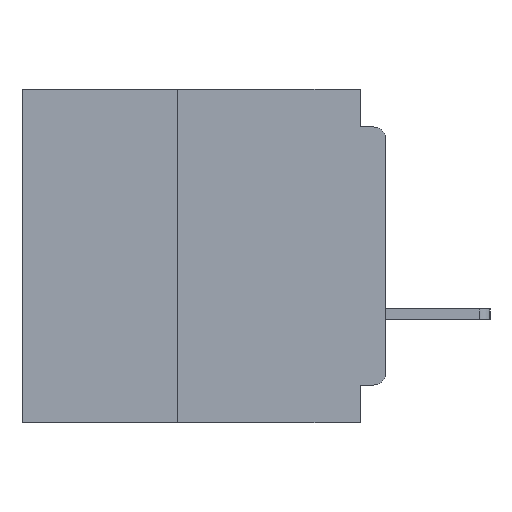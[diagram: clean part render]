
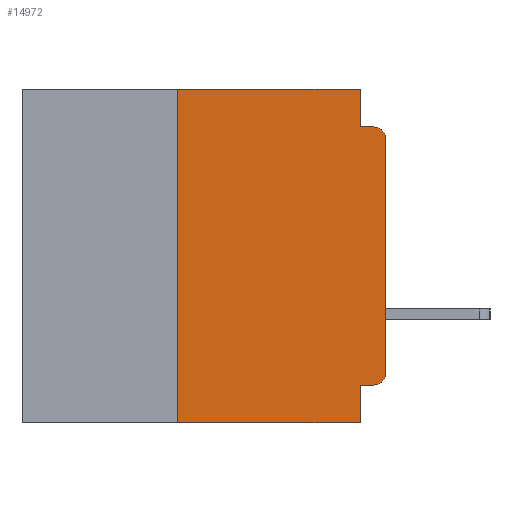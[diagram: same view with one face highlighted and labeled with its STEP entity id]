
A CAD part, left-side view. The second image highlights one B-rep face of the part: STEP entity #14972.
In plain terms, the highlighted planar face has unit normal (-1, 0, 0).
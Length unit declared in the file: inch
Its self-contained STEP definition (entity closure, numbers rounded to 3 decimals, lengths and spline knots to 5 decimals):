
#317 = ORIENTED_EDGE ( 'NONE', *, *, #792, .F. ) ;
#404 = CARTESIAN_POINT ( 'NONE',  ( 0., 0., -0.045 ) ) ;
#477 = LINE ( 'NONE', #39365, #16300 ) ;
#792 = EDGE_CURVE ( 'NONE', #34249, #23043, #32189, .T. ) ;
#835 = LINE ( 'NONE', #26741, #16669 ) ;
#1063 = ORIENTED_EDGE ( 'NONE', *, *, #35145, .T. ) ;
#1372 = LINE ( 'NONE', #39478, #8784 ) ;
#1627 = CARTESIAN_POINT ( 'NONE',  ( 0., 0.25, -0.4 ) ) ;
#2111 = DIRECTION ( 'NONE',  ( 0., 0., -1. ) ) ;
#2908 = EDGE_CURVE ( 'NONE', #33924, #28827, #24180, .T. ) ;
#3327 = CARTESIAN_POINT ( 'NONE',  ( 0., 0.031, -0.045 ) ) ;
#3510 = EDGE_CURVE ( 'NONE', #23043, #33924, #477, .T. ) ;
#3692 = ORIENTED_EDGE ( 'NONE', *, *, #33052, .F. ) ;
#4045 = ORIENTED_EDGE ( 'NONE', *, *, #2908, .F. ) ;
#4411 = DIRECTION ( 'NONE',  ( 1., 0., 0. ) ) ;
#4906 = DIRECTION ( 'NONE',  ( 0., 0., -1. ) ) ;
#4947 = ORIENTED_EDGE ( 'NONE', *, *, #22686, .F. ) ;
#4999 = EDGE_CURVE ( 'NONE', #9444, #7783, #835, .T. ) ;
#5172 = EDGE_LOOP ( 'NONE', ( #27229, #22282, #9449, #4045, #31001, #317, #1063, #3692, #4947, #5655 ) ) ;
#5655 = ORIENTED_EDGE ( 'NONE', *, *, #37965, .T. ) ;
#5801 = EDGE_CURVE ( 'NONE', #7783, #9494, #13127, .T. ) ;
#6443 = LINE ( 'NONE', #23766, #39601 ) ;
#7588 = CARTESIAN_POINT ( 'NONE',  ( 0., 0.031, -0.355 ) ) ;
#7783 = VERTEX_POINT ( 'NONE', #21004 ) ;
#8784 = VECTOR ( 'NONE', #24107, 39.37008 ) ;
#9444 = VERTEX_POINT ( 'NONE', #35533 ) ;
#9449 = ORIENTED_EDGE ( 'NONE', *, *, #37206, .F. ) ;
#9494 = VERTEX_POINT ( 'NONE', #26444 ) ;
#9513 = DIRECTION ( 'NONE',  ( 0., 0., -1. ) ) ;
#9569 = DIRECTION ( 'NONE',  ( -1., 0., 0. ) ) ;
#9646 = CARTESIAN_POINT ( 'NONE',  ( 0., 0.015, -0.06 ) ) ;
#12024 = VECTOR ( 'NONE', #18635, 39.37008 ) ;
#13127 = CIRCLE ( 'NONE', #31725, 0.015 ) ;
#14162 = CARTESIAN_POINT ( 'NONE',  ( 0., 0.25, 0. ) ) ;
#14673 = AXIS2_PLACEMENT_3D ( 'NONE', #23292, #4411, #26365 ) ;
#14972 = ADVANCED_FACE ( 'NONE', ( #22209 ), #35587, .F. ) ;
#15386 = VERTEX_POINT ( 'NONE', #32702 ) ;
#15880 = VECTOR ( 'NONE', #22164, 39.37008 ) ;
#16168 = DIRECTION ( 'NONE',  ( 0., -1., 0. ) ) ;
#16300 = VECTOR ( 'NONE', #39157, 39.37008 ) ;
#16549 = DIRECTION ( 'NONE',  ( 0., 0., 1. ) ) ;
#16669 = VECTOR ( 'NONE', #26215, 39.37008 ) ;
#18253 = CARTESIAN_POINT ( 'NONE',  ( 0., 0.015, -0.355 ) ) ;
#18635 = DIRECTION ( 'NONE',  ( 0., 1., 0. ) ) ;
#20461 = LINE ( 'NONE', #30924, #12024 ) ;
#21004 = CARTESIAN_POINT ( 'NONE',  ( 0., 0., -0.06 ) ) ;
#21076 = DIRECTION ( 'NONE',  ( -1., 0., 0. ) ) ;
#22164 = DIRECTION ( 'NONE',  ( 0., 0., -1. ) ) ;
#22209 = FACE_OUTER_BOUND ( 'NONE', #5172, .T. ) ;
#22282 = ORIENTED_EDGE ( 'NONE', *, *, #5801, .T. ) ;
#22686 = EDGE_CURVE ( 'NONE', #29262, #24522, #20461, .T. ) ;
#23043 = VERTEX_POINT ( 'NONE', #14162 ) ;
#23167 = CARTESIAN_POINT ( 'NONE',  ( 0., 0.031, 0. ) ) ;
#23292 = CARTESIAN_POINT ( 'NONE',  ( 0., 0.437, 0. ) ) ;
#23766 = CARTESIAN_POINT ( 'NONE',  ( 0., 0.031, -0.4 ) ) ;
#24107 = DIRECTION ( 'NONE',  ( 0., -1., 0. ) ) ;
#24180 = LINE ( 'NONE', #23167, #15880 ) ;
#24522 = VERTEX_POINT ( 'NONE', #7588 ) ;
#26215 = DIRECTION ( 'NONE',  ( 0., 0., 1. ) ) ;
#26365 = DIRECTION ( 'NONE',  ( 0., 0., -1. ) ) ;
#26444 = CARTESIAN_POINT ( 'NONE',  ( 0., 0.015, -0.045 ) ) ;
#26741 = CARTESIAN_POINT ( 'NONE',  ( 0., 0., 0. ) ) ;
#27229 = ORIENTED_EDGE ( 'NONE', *, *, #4999, .T. ) ;
#27823 = AXIS2_PLACEMENT_3D ( 'NONE', #39505, #21076, #2111 ) ;
#28827 = VERTEX_POINT ( 'NONE', #3327 ) ;
#29262 = VERTEX_POINT ( 'NONE', #18253 ) ;
#29907 = CARTESIAN_POINT ( 'NONE',  ( 0., 0.25, -0.4 ) ) ;
#30536 = VECTOR ( 'NONE', #16168, 39.37008 ) ;
#30924 = CARTESIAN_POINT ( 'NONE',  ( 0., 0., -0.355 ) ) ;
#31001 = ORIENTED_EDGE ( 'NONE', *, *, #3510, .F. ) ;
#31240 = VECTOR ( 'NONE', #16549, 39.37008 ) ;
#31725 = AXIS2_PLACEMENT_3D ( 'NONE', #9646, #9569, #9513 ) ;
#32189 = LINE ( 'NONE', #1627, #31240 ) ;
#32702 = CARTESIAN_POINT ( 'NONE',  ( 0., 0.031, -0.4 ) ) ;
#33052 = EDGE_CURVE ( 'NONE', #24522, #15386, #6443, .T. ) ;
#33923 = CIRCLE ( 'NONE', #27823, 0.015 ) ;
#33924 = VERTEX_POINT ( 'NONE', #40155 ) ;
#34249 = VERTEX_POINT ( 'NONE', #29907 ) ;
#35145 = EDGE_CURVE ( 'NONE', #34249, #15386, #1372, .T. ) ;
#35533 = CARTESIAN_POINT ( 'NONE',  ( 0., 0., -0.34 ) ) ;
#35587 = PLANE ( 'NONE',  #14673 ) ;
#37206 = EDGE_CURVE ( 'NONE', #28827, #9494, #39691, .T. ) ;
#37965 = EDGE_CURVE ( 'NONE', #29262, #9444, #33923, .T. ) ;
#39157 = DIRECTION ( 'NONE',  ( 0., -1., 0. ) ) ;
#39365 = CARTESIAN_POINT ( 'NONE',  ( 0., 0.437, 0. ) ) ;
#39478 = CARTESIAN_POINT ( 'NONE',  ( 0., 0.437, -0.4 ) ) ;
#39505 = CARTESIAN_POINT ( 'NONE',  ( 0., 0.015, -0.34 ) ) ;
#39601 = VECTOR ( 'NONE', #4906, 39.37008 ) ;
#39691 = LINE ( 'NONE', #404, #30536 ) ;
#40155 = CARTESIAN_POINT ( 'NONE',  ( 0., 0.031, 0. ) ) ;
